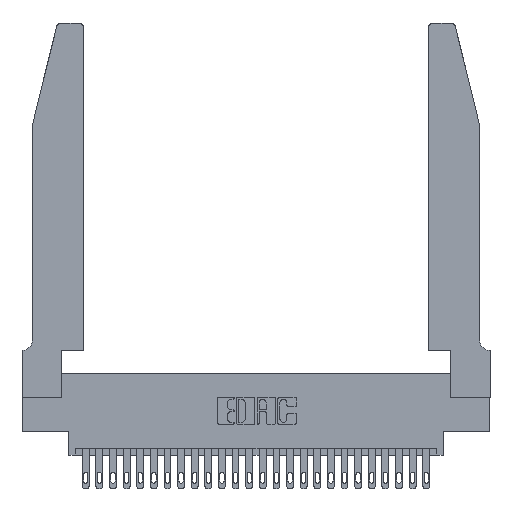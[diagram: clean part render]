
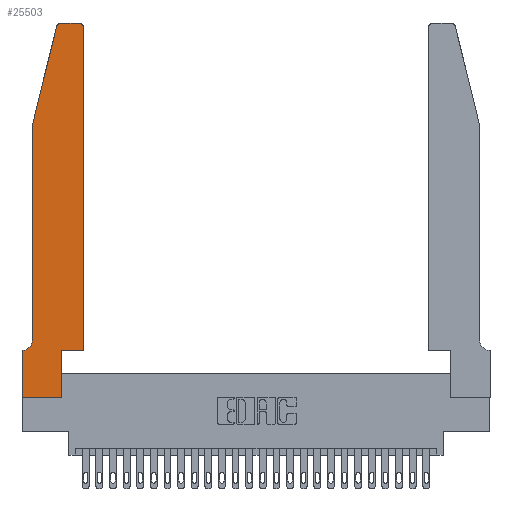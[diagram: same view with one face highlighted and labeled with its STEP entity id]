
A CAD part, top view. The second image highlights one B-rep face of the part: STEP entity #25503.
In plain terms, the highlighted planar face has unit normal (0, 0, 1).
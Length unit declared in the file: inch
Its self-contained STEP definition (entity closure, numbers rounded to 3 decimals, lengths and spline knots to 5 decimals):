
#355 = DIRECTION ( 'NONE',  ( 0., -1., 0. ) ) ;
#356 = DIRECTION ( 'NONE',  ( 0., -1., 0. ) ) ;
#632 = DIRECTION ( 'NONE',  ( 0., 0., 1. ) ) ;
#1014 = VERTEX_POINT ( 'NONE', #2849 ) ;
#1064 = CARTESIAN_POINT ( 'NONE',  ( 0.0755, 2., 0.37 ) ) ;
#1075 = ORIENTED_EDGE ( 'NONE', *, *, #10619, .T. ) ;
#1096 = VERTEX_POINT ( 'NONE', #1945 ) ;
#1160 = ORIENTED_EDGE ( 'NONE', *, *, #22454, .T. ) ;
#1511 = VECTOR ( 'NONE', #5813, 39.37008 ) ;
#1546 = ORIENTED_EDGE ( 'NONE', *, *, #6047, .T. ) ;
#1795 = VERTEX_POINT ( 'NONE', #14809 ) ;
#1945 = CARTESIAN_POINT ( 'NONE',  ( 0.2865, 0.35, 0.37 ) ) ;
#2238 = EDGE_CURVE ( 'NONE', #22221, #1795, #3962, .T. ) ;
#2478 = CARTESIAN_POINT ( 'NONE',  ( 0.4505, 0.35, 0.37 ) ) ;
#2716 = EDGE_CURVE ( 'NONE', #10755, #17415, #18505, .T. ) ;
#2849 = CARTESIAN_POINT ( 'NONE',  ( 0., 0.35, 0.37 ) ) ;
#2883 = FACE_OUTER_BOUND ( 'NONE', #16473, .T. ) ;
#3270 = VECTOR ( 'NONE', #19363, 39.37008 ) ;
#3676 = VECTOR ( 'NONE', #15788, 39.37008 ) ;
#3962 = LINE ( 'NONE', #7210, #13249 ) ;
#4028 = VERTEX_POINT ( 'NONE', #6696 ) ;
#4547 = CARTESIAN_POINT ( 'NONE',  ( 0.284, 2.72, 0.37 ) ) ;
#4947 = EDGE_CURVE ( 'NONE', #19970, #14157, #25606, .T. ) ;
#5022 = AXIS2_PLACEMENT_3D ( 'NONE', #4547, #632, #8753 ) ;
#5060 = CIRCLE ( 'NONE', #6218, 0.07 ) ;
#5147 = VECTOR ( 'NONE', #13576, 39.37008 ) ;
#5748 = VECTOR ( 'NONE', #9813, 39.37008 ) ;
#5813 = DIRECTION ( 'NONE',  ( 0., 1., 0. ) ) ;
#5940 = CARTESIAN_POINT ( 'NONE',  ( 0.0755, 2., 0.37 ) ) ;
#5999 = LINE ( 'NONE', #13715, #3676 ) ;
#6047 = EDGE_CURVE ( 'NONE', #18440, #1014, #26094, .T. ) ;
#6218 = AXIS2_PLACEMENT_3D ( 'NONE', #24798, #12215, #14046 ) ;
#6232 = CARTESIAN_POINT ( 'NONE',  ( 0.284, 2.75, 0.37 ) ) ;
#6696 = CARTESIAN_POINT ( 'NONE',  ( 0.4505, 0.35, 0.37 ) ) ;
#7210 = CARTESIAN_POINT ( 'NONE',  ( 0., 0., 0.37 ) ) ;
#8753 = DIRECTION ( 'NONE',  ( 1., 0., 0. ) ) ;
#8944 = VERTEX_POINT ( 'NONE', #6232 ) ;
#9768 = ORIENTED_EDGE ( 'NONE', *, *, #17910, .T. ) ;
#9813 = DIRECTION ( 'NONE',  ( 1., 0., 0. ) ) ;
#9915 = CARTESIAN_POINT ( 'NONE',  ( 0.4205, 2.75, 0.37 ) ) ;
#10619 = EDGE_CURVE ( 'NONE', #1096, #4028, #23881, .T. ) ;
#10719 = CIRCLE ( 'NONE', #5022, 0.03 ) ;
#10755 = VERTEX_POINT ( 'NONE', #25134 ) ;
#10897 = DIRECTION ( 'NONE',  ( 1., 0., 0. ) ) ;
#11105 = CARTESIAN_POINT ( 'NONE',  ( 0.0755, 0.35, 0.37 ) ) ;
#11203 = CARTESIAN_POINT ( 'NONE',  ( 0., 0., 0.37 ) ) ;
#11642 = CARTESIAN_POINT ( 'NONE',  ( 0.0755, 2., 0.37 ) ) ;
#11688 = DIRECTION ( 'NONE',  ( 1., 0., 0. ) ) ;
#11724 = EDGE_CURVE ( 'NONE', #1795, #1096, #5999, .T. ) ;
#11834 = EDGE_CURVE ( 'NONE', #1014, #22221, #14935, .T. ) ;
#11880 = EDGE_CURVE ( 'NONE', #17415, #8944, #16251, .T. ) ;
#12140 = CARTESIAN_POINT ( 'NONE',  ( 0.4505, 0.35, 0.37 ) ) ;
#12215 = DIRECTION ( 'NONE',  ( 0., 0., -1. ) ) ;
#12487 = LINE ( 'NONE', #12140, #1511 ) ;
#13032 = EDGE_CURVE ( 'NONE', #8944, #19970, #10719, .T. ) ;
#13098 = VECTOR ( 'NONE', #356, 39.37008 ) ;
#13249 = VECTOR ( 'NONE', #11688, 39.37008 ) ;
#13576 = DIRECTION ( 'NONE',  ( -0.239, -0.971, 0. ) ) ;
#13715 = CARTESIAN_POINT ( 'NONE',  ( 0.2865, 0.35, 0.37 ) ) ;
#14046 = DIRECTION ( 'NONE',  ( -1., 0., 0. ) ) ;
#14157 = VERTEX_POINT ( 'NONE', #5940 ) ;
#14799 = ORIENTED_EDGE ( 'NONE', *, *, #4947, .T. ) ;
#14809 = CARTESIAN_POINT ( 'NONE',  ( 0.2865, 0., 0.37 ) ) ;
#14935 = LINE ( 'NONE', #22224, #25460 ) ;
#15589 = VECTOR ( 'NONE', #24988, 39.37008 ) ;
#15788 = DIRECTION ( 'NONE',  ( 0., 1., 0. ) ) ;
#16251 = LINE ( 'NONE', #27111, #15589 ) ;
#16473 = EDGE_LOOP ( 'NONE', ( #22713, #24282, #14799, #9768, #1160, #1546, #18105, #20361, #20198, #1075, #19633, #26597 ) ) ;
#16551 = VERTEX_POINT ( 'NONE', #22834 ) ;
#16553 = AXIS2_PLACEMENT_3D ( 'NONE', #24573, #17837, #22682 ) ;
#17306 = CARTESIAN_POINT ( 'NONE',  ( 0.0055, 0.35, 0.37 ) ) ;
#17415 = VERTEX_POINT ( 'NONE', #9915 ) ;
#17578 = EDGE_CURVE ( 'NONE', #4028, #10755, #12487, .T. ) ;
#17837 = DIRECTION ( 'NONE',  ( 0., 0., 1. ) ) ;
#17910 = EDGE_CURVE ( 'NONE', #14157, #16551, #26925, .T. ) ;
#18105 = ORIENTED_EDGE ( 'NONE', *, *, #11834, .T. ) ;
#18440 = VERTEX_POINT ( 'NONE', #17306 ) ;
#18505 = CIRCLE ( 'NONE', #16553, 0.03 ) ;
#19363 = DIRECTION ( 'NONE',  ( -1., 0., 0. ) ) ;
#19633 = ORIENTED_EDGE ( 'NONE', *, *, #17578, .T. ) ;
#19970 = VERTEX_POINT ( 'NONE', #21032 ) ;
#20198 = ORIENTED_EDGE ( 'NONE', *, *, #11724, .T. ) ;
#20361 = ORIENTED_EDGE ( 'NONE', *, *, #2238, .T. ) ;
#21032 = CARTESIAN_POINT ( 'NONE',  ( 0.25487, 2.72718, 0.37 ) ) ;
#21357 = DIRECTION ( 'NONE',  ( 0., 0., 1. ) ) ;
#22221 = VERTEX_POINT ( 'NONE', #11203 ) ;
#22224 = CARTESIAN_POINT ( 'NONE',  ( 0., 0., 0.37 ) ) ;
#22454 = EDGE_CURVE ( 'NONE', #16551, #18440, #5060, .T. ) ;
#22682 = DIRECTION ( 'NONE',  ( 1., 0., 0. ) ) ;
#22713 = ORIENTED_EDGE ( 'NONE', *, *, #11880, .T. ) ;
#22834 = CARTESIAN_POINT ( 'NONE',  ( 0.0755, 0.42, 0.37 ) ) ;
#23570 = CARTESIAN_POINT ( 'NONE',  ( 0., 0.35, 0.37 ) ) ;
#23881 = LINE ( 'NONE', #2478, #5748 ) ;
#24282 = ORIENTED_EDGE ( 'NONE', *, *, #13032, .T. ) ;
#24573 = CARTESIAN_POINT ( 'NONE',  ( 0.4205, 2.72, 0.37 ) ) ;
#24798 = CARTESIAN_POINT ( 'NONE',  ( 0.0055, 0.42, 0.37 ) ) ;
#24988 = DIRECTION ( 'NONE',  ( -1., 0., 0. ) ) ;
#25134 = CARTESIAN_POINT ( 'NONE',  ( 0.4505, 2.72, 0.37 ) ) ;
#25324 = PLANE ( 'NONE',  #25676 ) ;
#25460 = VECTOR ( 'NONE', #355, 39.37008 ) ;
#25503 = ADVANCED_FACE ( 'NONE', ( #2883 ), #25324, .T. ) ;
#25606 = LINE ( 'NONE', #11642, #5147 ) ;
#25676 = AXIS2_PLACEMENT_3D ( 'NONE', #23570, #21357, #10897 ) ;
#26094 = LINE ( 'NONE', #11105, #3270 ) ;
#26597 = ORIENTED_EDGE ( 'NONE', *, *, #2716, .T. ) ;
#26925 = LINE ( 'NONE', #1064, #13098 ) ;
#27111 = CARTESIAN_POINT ( 'NONE',  ( 0.2605, 2.75, 0.37 ) ) ;
